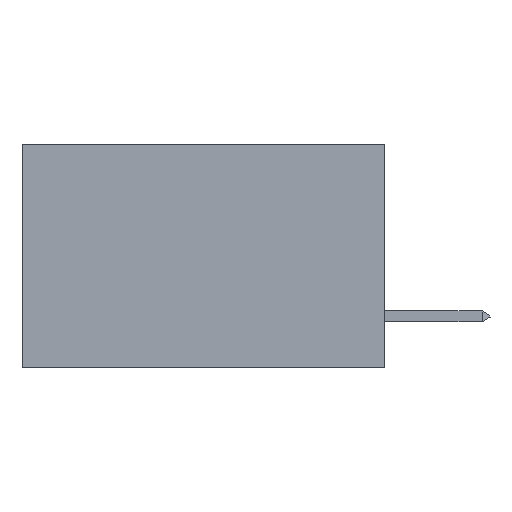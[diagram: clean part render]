
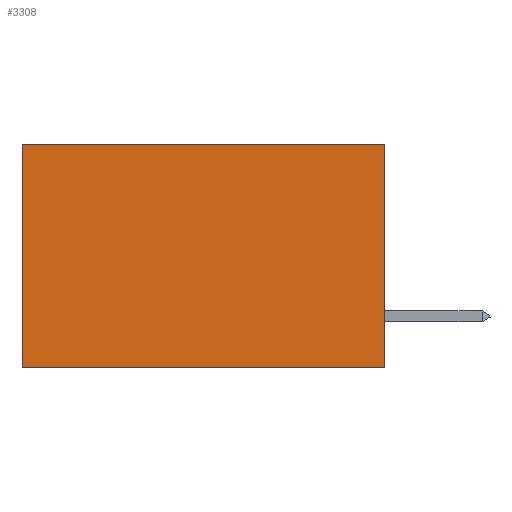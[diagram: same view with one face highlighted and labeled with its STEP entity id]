
A CAD part, left-side view. The second image highlights one B-rep face of the part: STEP entity #3308.
In plain terms, the highlighted planar face has unit normal (-1, 0, 0).
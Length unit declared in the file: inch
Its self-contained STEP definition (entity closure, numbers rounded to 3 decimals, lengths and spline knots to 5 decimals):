
#329 = FACE_OUTER_BOUND ( 'NONE', #2027, .T. ) ;
#778 = VECTOR ( 'NONE', #6294, 39.37008 ) ;
#1572 = AXIS2_PLACEMENT_3D ( 'NONE', #3040, #15221, #13697 ) ;
#1614 = DIRECTION ( 'NONE',  ( 0., 0., -1. ) ) ;
#1673 = CARTESIAN_POINT ( 'NONE',  ( 0.2875, 0., -0.37 ) ) ;
#1684 = EDGE_CURVE ( 'NONE', #14353, #2281, #16826, .T. ) ;
#1940 = CARTESIAN_POINT ( 'NONE',  ( 0.2875, 0., -0.37 ) ) ;
#2027 = EDGE_LOOP ( 'NONE', ( #13947, #9452, #3640, #12199 ) ) ;
#2281 = VERTEX_POINT ( 'NONE', #16760 ) ;
#2907 = CARTESIAN_POINT ( 'NONE',  ( 0.2875, 0.6, -0.37 ) ) ;
#2955 = VECTOR ( 'NONE', #7694, 39.37008 ) ;
#3040 = CARTESIAN_POINT ( 'NONE',  ( 0.2875, 0., 0. ) ) ;
#3308 = ADVANCED_FACE ( 'NONE', ( #329 ), #14959, .F. ) ;
#3640 = ORIENTED_EDGE ( 'NONE', *, *, #3722, .F. ) ;
#3722 = EDGE_CURVE ( 'NONE', #14353, #14726, #18850, .T. ) ;
#3751 = EDGE_CURVE ( 'NONE', #2281, #11246, #17193, .T. ) ;
#4488 = CARTESIAN_POINT ( 'NONE',  ( 0.2875, 0.6, 0. ) ) ;
#6294 = DIRECTION ( 'NONE',  ( 0., 1., 0. ) ) ;
#7694 = DIRECTION ( 'NONE',  ( 0., 0., -1. ) ) ;
#9452 = ORIENTED_EDGE ( 'NONE', *, *, #10270, .F. ) ;
#10270 = EDGE_CURVE ( 'NONE', #14726, #11246, #18613, .T. ) ;
#10402 = DIRECTION ( 'NONE',  ( 0., 1., 0. ) ) ;
#10706 = CARTESIAN_POINT ( 'NONE',  ( 0.2875, 0., 0. ) ) ;
#11246 = VERTEX_POINT ( 'NONE', #2907 ) ;
#12199 = ORIENTED_EDGE ( 'NONE', *, *, #1684, .T. ) ;
#13190 = VECTOR ( 'NONE', #1614, 39.37008 ) ;
#13697 = DIRECTION ( 'NONE',  ( 0., 0., -1. ) ) ;
#13947 = ORIENTED_EDGE ( 'NONE', *, *, #3751, .T. ) ;
#14353 = VERTEX_POINT ( 'NONE', #10706 ) ;
#14726 = VERTEX_POINT ( 'NONE', #1673 ) ;
#14911 = CARTESIAN_POINT ( 'NONE',  ( 0.2875, 0., 0. ) ) ;
#14959 = PLANE ( 'NONE',  #1572 ) ;
#15221 = DIRECTION ( 'NONE',  ( 1., 0., 0. ) ) ;
#16760 = CARTESIAN_POINT ( 'NONE',  ( 0.2875, 0.6, 0. ) ) ;
#16826 = LINE ( 'NONE', #14911, #18470 ) ;
#17193 = LINE ( 'NONE', #4488, #13190 ) ;
#18470 = VECTOR ( 'NONE', #10402, 39.37008 ) ;
#18613 = LINE ( 'NONE', #1940, #778 ) ;
#18850 = LINE ( 'NONE', #19552, #2955 ) ;
#19552 = CARTESIAN_POINT ( 'NONE',  ( 0.2875, 0., 0. ) ) ;
